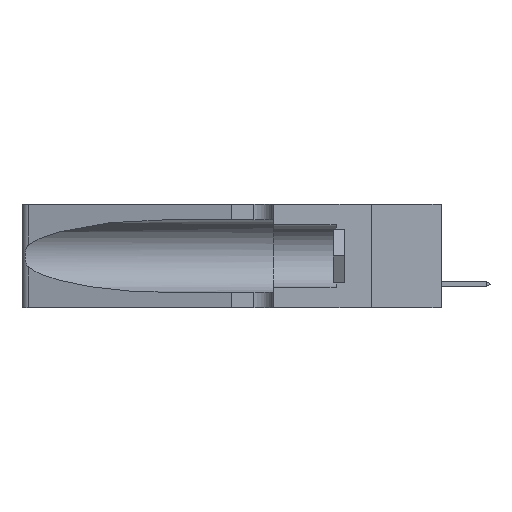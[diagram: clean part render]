
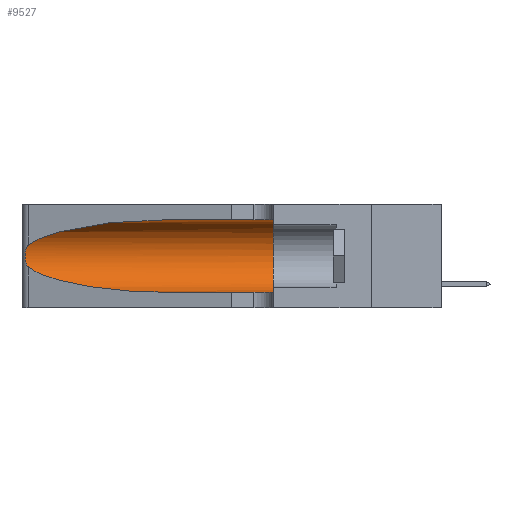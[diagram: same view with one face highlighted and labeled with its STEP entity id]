
A CAD part, left-side view. The second image highlights one B-rep face of the part: STEP entity #9527.
In plain terms, the highlighted cylindrical face has radius 3.308 mm (diameter 6.617 mm), a partial arc.
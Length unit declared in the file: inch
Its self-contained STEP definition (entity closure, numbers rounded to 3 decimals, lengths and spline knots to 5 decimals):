
#431 = CARTESIAN_POINT ( 'NONE',  ( 0.1305, 0.72297, 0.05475 ) ) ;
#521 = CARTESIAN_POINT ( 'NONE',  ( 0.1305, 0.72297, 0.31525 ) ) ;
#1186 = AXIS2_PLACEMENT_3D ( 'NONE', #14810, #6540, #16197 ) ;
#1198 = DIRECTION ( 'NONE',  ( 0., -1., 0. ) ) ;
#1514 = CARTESIAN_POINT ( 'NONE',  ( 0.26018, 1.23835, 0.19895 ) ) ;
#1573 = CARTESIAN_POINT ( 'NONE',  ( 0.26017, 1.23833, 0.17102 ) ) ;
#1900 = CARTESIAN_POINT ( 'NONE',  ( 0.18966, 0.96281, 0.05475 ) ) ;
#2421 = CARTESIAN_POINT ( 'NONE',  ( 0.1305, 1.61858, 0.05475 ) ) ;
#2574 = CARTESIAN_POINT ( 'NONE',  ( 0.18966, 0.96281, 0.31525 ) ) ;
#2877 = EDGE_CURVE ( 'NONE', #16383, #15576, #15767, .T. ) ;
#3096 = EDGE_LOOP ( 'NONE', ( #10021, #12407, #12216, #8998, #10593, #9888 ) ) ;
#3174 = CARTESIAN_POINT ( 'NONE',  ( 0.25555, 1.22993, 0.14849 ) ) ;
#3979 = EDGE_CURVE ( 'NONE', #9618, #13317, #10034, .T. ) ;
#4276 = CARTESIAN_POINT ( 'NONE',  ( 0.26075, 1.23896, 0.19203 ) ) ;
#4441 = CARTESIAN_POINT ( 'NONE',  ( 0.2373, 1.15595, 0.08982 ) ) ;
#4577 = CARTESIAN_POINT ( 'NONE',  ( 0.25487, 1.22718, 0.14631 ) ) ;
#4694 = CARTESIAN_POINT ( 'NONE',  ( 0.25487, 1.22718, 0.14631 ) ) ;
#4705 = EDGE_CURVE ( 'NONE', #16383, #9618, #16628, .T. ) ;
#5313 = CARTESIAN_POINT ( 'NONE',  ( 0.25487, 1.22718, 0.22369 ) ) ;
#5427 = CARTESIAN_POINT ( 'NONE',  ( 0.2373, 1.15595, 0.28018 ) ) ;
#5677 = CARTESIAN_POINT ( 'NONE',  ( 0.26075, 1.23896, 0.178 ) ) ;
#6315 = DIRECTION ( 'NONE',  ( 0., -1., 0. ) ) ;
#6371 = DIRECTION ( 'NONE',  ( 0., 0., -1. ) ) ;
#6540 = DIRECTION ( 'NONE',  ( 0., 1., 0. ) ) ;
#6982 = CARTESIAN_POINT ( 'NONE',  ( 0.25787, 1.23484, 0.2124 ) ) ;
#7652 = CARTESIAN_POINT ( 'NONE',  ( 0.1305, 0.35, 0.31525 ) ) ;
#7687 = CARTESIAN_POINT ( 'NONE',  ( 0.1305, 0.35, 0.05475 ) ) ;
#8348 = VERTEX_POINT ( 'NONE', #4694 ) ;
#8998 = ORIENTED_EDGE ( 'NONE', *, *, #9121, .T. ) ;
#9063 = CARTESIAN_POINT ( 'NONE',  ( 0.25487, 1.22718, 0.22369 ) ) ;
#9121 = EDGE_CURVE ( 'NONE', #10019, #13317, #15802, .T. ) ;
#9527 = ADVANCED_FACE ( 'NONE', ( #9744 ), #16471, .F. ) ;
#9618 = VERTEX_POINT ( 'NONE', #7652 ) ;
#9676 =( BOUNDED_CURVE ( )  B_SPLINE_CURVE ( 3, ( #15536, #4441, #1900, #431 ),
 .UNSPECIFIED., .F., .F. ) 
 B_SPLINE_CURVE_WITH_KNOTS ( ( 4, 4 ),
 ( 3.44316, 4.71239 ),
 .UNSPECIFIED. ) 
 CURVE ( )  GEOMETRIC_REPRESENTATION_ITEM ( )  RATIONAL_B_SPLINE_CURVE ( ( 1., 0.87, 0.87, 1. ) ) 
 REPRESENTATION_ITEM ( '' )  );
#9744 = FACE_OUTER_BOUND ( 'NONE', #3096, .T. ) ;
#9759 = CARTESIAN_POINT ( 'NONE',  ( 0.25854, 1.2359, 0.20912 ) ) ;
#9812 = CARTESIAN_POINT ( 'NONE',  ( 0.25639, 1.23184, 0.21858 ) ) ;
#9888 = ORIENTED_EDGE ( 'NONE', *, *, #4705, .F. ) ;
#9986 = CARTESIAN_POINT ( 'NONE',  ( 0.25487, 1.22718, 0.22369 ) ) ;
#10019 = VERTEX_POINT ( 'NONE', #14203 ) ;
#10021 = ORIENTED_EDGE ( 'NONE', *, *, #2877, .T. ) ;
#10034 = CIRCLE ( 'NONE', #1186, 0.13025 ) ;
#10593 = ORIENTED_EDGE ( 'NONE', *, *, #3979, .F. ) ;
#11430 = CARTESIAN_POINT ( 'NONE',  ( 0.25789, 1.23486, 0.15765 ) ) ;
#11559 = B_SPLINE_CURVE_WITH_KNOTS ( 'NONE', 3,
 ( #9986, #13851, #9812, #6982, #9759, #1514, #4276, #5677, #1573, #12599, #11430, #17116, #3174, #4577 ),
 .UNSPECIFIED., .F., .F.,
 ( 4, 2, 2, 2, 2, 2, 4 ),
 ( 0., 0.00027, 0.00053, 0.00107, 0.0016, 0.00187, 0.00214 ),
 .UNSPECIFIED. ) ;
#12216 = ORIENTED_EDGE ( 'NONE', *, *, #16799, .T. ) ;
#12407 = ORIENTED_EDGE ( 'NONE', *, *, #12847, .T. ) ;
#12599 = CARTESIAN_POINT ( 'NONE',  ( 0.25856, 1.23593, 0.16098 ) ) ;
#12616 = CARTESIAN_POINT ( 'NONE',  ( 0.1305, 1.61858, 0.31525 ) ) ;
#12847 = EDGE_CURVE ( 'NONE', #15576, #8348, #11559, .T. ) ;
#12950 = VECTOR ( 'NONE', #15564, 39.37008 ) ;
#13317 = VERTEX_POINT ( 'NONE', #7687 ) ;
#13545 = CARTESIAN_POINT ( 'NONE',  ( 0.1305, 0.72297, 0.31525 ) ) ;
#13648 = VECTOR ( 'NONE', #1198, 39.37008 ) ;
#13851 = CARTESIAN_POINT ( 'NONE',  ( 0.25555, 1.22994, 0.2215 ) ) ;
#14203 = CARTESIAN_POINT ( 'NONE',  ( 0.1305, 0.72297, 0.05475 ) ) ;
#14810 = CARTESIAN_POINT ( 'NONE',  ( 0.1305, 0.35, 0.185 ) ) ;
#15536 = CARTESIAN_POINT ( 'NONE',  ( 0.25487, 1.22718, 0.14631 ) ) ;
#15564 = DIRECTION ( 'NONE',  ( 0., -1., 0. ) ) ;
#15576 = VERTEX_POINT ( 'NONE', #9063 ) ;
#15767 =( BOUNDED_CURVE ( )  B_SPLINE_CURVE ( 3, ( #13545, #2574, #5427, #5313 ),
 .UNSPECIFIED., .F., .F. ) 
 B_SPLINE_CURVE_WITH_KNOTS ( ( 4, 4 ),
 ( 1.5708, 2.84003 ),
 .UNSPECIFIED. ) 
 CURVE ( )  GEOMETRIC_REPRESENTATION_ITEM ( )  RATIONAL_B_SPLINE_CURVE ( ( 1., 0.87, 0.87, 1. ) ) 
 REPRESENTATION_ITEM ( '' )  );
#15802 = LINE ( 'NONE', #2421, #13648 ) ;
#15961 = CARTESIAN_POINT ( 'NONE',  ( 0.1305, 1.61858, 0.185 ) ) ;
#16087 = AXIS2_PLACEMENT_3D ( 'NONE', #15961, #6315, #6371 ) ;
#16197 = DIRECTION ( 'NONE',  ( 0., 0., 1. ) ) ;
#16383 = VERTEX_POINT ( 'NONE', #521 ) ;
#16471 = CYLINDRICAL_SURFACE ( 'NONE', #16087, 0.13025 ) ;
#16628 = LINE ( 'NONE', #12616, #12950 ) ;
#16799 = EDGE_CURVE ( 'NONE', #8348, #10019, #9676, .T. ) ;
#17116 = CARTESIAN_POINT ( 'NONE',  ( 0.25639, 1.23186, 0.15144 ) ) ;
